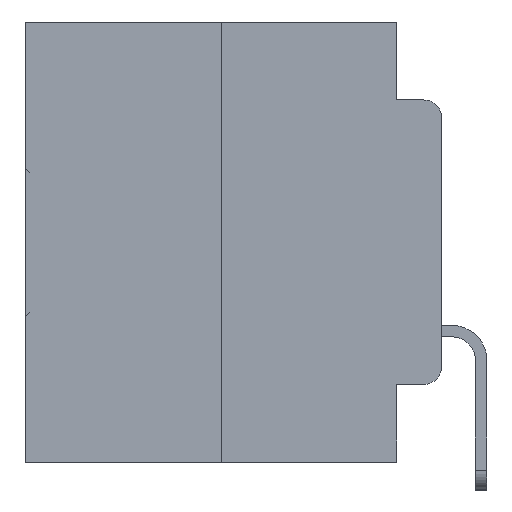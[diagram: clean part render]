
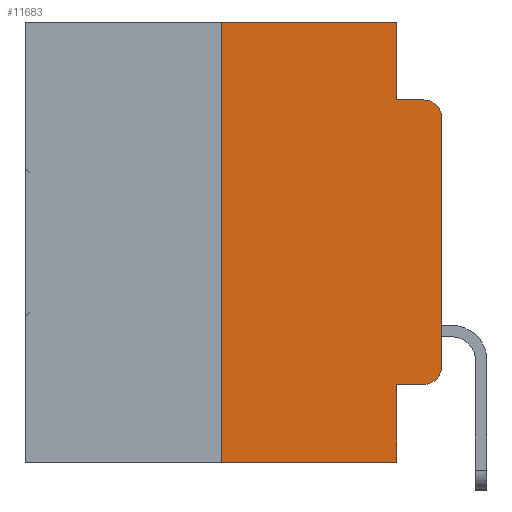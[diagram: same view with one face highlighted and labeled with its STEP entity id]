
A CAD part, left-side view. The second image highlights one B-rep face of the part: STEP entity #11683.
In plain terms, the highlighted planar face has unit normal (-1, 0, 0).
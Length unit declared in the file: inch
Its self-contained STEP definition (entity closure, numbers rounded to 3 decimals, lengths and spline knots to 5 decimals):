
#506 = CARTESIAN_POINT ( 'NONE',  ( 0., 0.473, -0.5 ) ) ;
#523 = LINE ( 'NONE', #14726, #13903 ) ;
#808 = CARTESIAN_POINT ( 'NONE',  ( 0., 0.051, -0.4115 ) ) ;
#1517 = CARTESIAN_POINT ( 'NONE',  ( 0., 0.473, 0. ) ) ;
#1550 = EDGE_CURVE ( 'NONE', #27723, #16165, #23982, .T. ) ;
#2521 = LINE ( 'NONE', #28439, #27292 ) ;
#3040 = CARTESIAN_POINT ( 'NONE',  ( 0., 0.051, 0. ) ) ;
#3444 = AXIS2_PLACEMENT_3D ( 'NONE', #1517, #19579, #4338 ) ;
#4338 = DIRECTION ( 'NONE',  ( 0., 0., -1. ) ) ;
#4409 = EDGE_LOOP ( 'NONE', ( #30576, #19176, #9866, #19543, #31645, #8665, #29174, #15020, #27448, #17326 ) ) ;
#4713 = VERTEX_POINT ( 'NONE', #7972 ) ;
#4995 = CARTESIAN_POINT ( 'NONE',  ( 0., 0.02, -0.1085 ) ) ;
#5951 = CARTESIAN_POINT ( 'NONE',  ( 0., 0., -0.1085 ) ) ;
#7069 = VERTEX_POINT ( 'NONE', #9125 ) ;
#7181 = DIRECTION ( 'NONE',  ( 0., 0., -1. ) ) ;
#7466 = CIRCLE ( 'NONE', #23512, 0.02 ) ;
#7744 = DIRECTION ( 'NONE',  ( 0., 0., -1. ) ) ;
#7972 = CARTESIAN_POINT ( 'NONE',  ( 0., 0.25, -0.5 ) ) ;
#8665 = ORIENTED_EDGE ( 'NONE', *, *, #12563, .F. ) ;
#9125 = CARTESIAN_POINT ( 'NONE',  ( 0., 0.051, -0.0885 ) ) ;
#9246 = DIRECTION ( 'NONE',  ( 0., -1., 0. ) ) ;
#9646 = VERTEX_POINT ( 'NONE', #808 ) ;
#9866 = ORIENTED_EDGE ( 'NONE', *, *, #18509, .F. ) ;
#11180 = VECTOR ( 'NONE', #24997, 39.37008 ) ;
#11683 = ADVANCED_FACE ( 'NONE', ( #27561 ), #26423, .F. ) ;
#11932 = LINE ( 'NONE', #506, #29934 ) ;
#12384 = CARTESIAN_POINT ( 'NONE',  ( 0., 0.051, -0.0885 ) ) ;
#12563 = EDGE_CURVE ( 'NONE', #4713, #16978, #14707, .T. ) ;
#12642 = CARTESIAN_POINT ( 'NONE',  ( 0., 0.02, -0.3915 ) ) ;
#13329 = CARTESIAN_POINT ( 'NONE',  ( 0., 0., -0.3915 ) ) ;
#13543 = VERTEX_POINT ( 'NONE', #19610 ) ;
#13674 = CIRCLE ( 'NONE', #15097, 0.02 ) ;
#13903 = VECTOR ( 'NONE', #17190, 39.37008 ) ;
#14136 = LINE ( 'NONE', #12384, #31931 ) ;
#14707 = LINE ( 'NONE', #27956, #26469 ) ;
#14726 = CARTESIAN_POINT ( 'NONE',  ( 0., 0.473, 0. ) ) ;
#14885 = DIRECTION ( 'NONE',  ( 0., -1., 0. ) ) ;
#14890 = CARTESIAN_POINT ( 'NONE',  ( 0., 0.051, 0. ) ) ;
#15020 = ORIENTED_EDGE ( 'NONE', *, *, #30381, .F. ) ;
#15097 = AXIS2_PLACEMENT_3D ( 'NONE', #4995, #22463, #7744 ) ;
#15130 = DIRECTION ( 'NONE',  ( 0., 0., -1. ) ) ;
#16165 = VERTEX_POINT ( 'NONE', #5951 ) ;
#16978 = VERTEX_POINT ( 'NONE', #28145 ) ;
#17190 = DIRECTION ( 'NONE',  ( 0., -1., 0. ) ) ;
#17326 = ORIENTED_EDGE ( 'NONE', *, *, #29039, .T. ) ;
#17896 = VERTEX_POINT ( 'NONE', #31397 ) ;
#18509 = EDGE_CURVE ( 'NONE', #7069, #19361, #14136, .T. ) ;
#19176 = ORIENTED_EDGE ( 'NONE', *, *, #22638, .T. ) ;
#19361 = VERTEX_POINT ( 'NONE', #31208 ) ;
#19543 = ORIENTED_EDGE ( 'NONE', *, *, #29808, .F. ) ;
#19579 = DIRECTION ( 'NONE',  ( 1., 0., 0. ) ) ;
#19610 = CARTESIAN_POINT ( 'NONE',  ( 0., 0.02, -0.4115 ) ) ;
#19657 = VERTEX_POINT ( 'NONE', #21021 ) ;
#20865 = DIRECTION ( 'NONE',  ( 0., 0., -1. ) ) ;
#21021 = CARTESIAN_POINT ( 'NONE',  ( 0., 0.051, -0.5 ) ) ;
#21140 = DIRECTION ( 'NONE',  ( 0., -1., 0. ) ) ;
#22463 = DIRECTION ( 'NONE',  ( -1., 0., 0. ) ) ;
#22638 = EDGE_CURVE ( 'NONE', #16165, #19361, #13674, .T. ) ;
#23369 = LINE ( 'NONE', #3040, #28646 ) ;
#23512 = AXIS2_PLACEMENT_3D ( 'NONE', #12642, #29044, #15130 ) ;
#23982 = LINE ( 'NONE', #24961, #11180 ) ;
#24854 = LINE ( 'NONE', #14890, #30791 ) ;
#24961 = CARTESIAN_POINT ( 'NONE',  ( 0., 0., 0. ) ) ;
#24997 = DIRECTION ( 'NONE',  ( 0., 0., 1. ) ) ;
#25490 = EDGE_CURVE ( 'NONE', #9646, #13543, #2521, .T. ) ;
#26423 = PLANE ( 'NONE',  #3444 ) ;
#26469 = VECTOR ( 'NONE', #30216, 39.37008 ) ;
#27292 = VECTOR ( 'NONE', #9246, 39.37008 ) ;
#27448 = ORIENTED_EDGE ( 'NONE', *, *, #25490, .T. ) ;
#27561 = FACE_OUTER_BOUND ( 'NONE', #4409, .T. ) ;
#27723 = VERTEX_POINT ( 'NONE', #13329 ) ;
#27956 = CARTESIAN_POINT ( 'NONE',  ( 0., 0.25, 0. ) ) ;
#28145 = CARTESIAN_POINT ( 'NONE',  ( 0., 0.25, 0. ) ) ;
#28229 = EDGE_CURVE ( 'NONE', #16978, #17896, #523, .T. ) ;
#28439 = CARTESIAN_POINT ( 'NONE',  ( 0., 0.051, -0.4115 ) ) ;
#28600 = EDGE_CURVE ( 'NONE', #4713, #19657, #11932, .T. ) ;
#28646 = VECTOR ( 'NONE', #20865, 39.37008 ) ;
#29039 = EDGE_CURVE ( 'NONE', #13543, #27723, #7466, .T. ) ;
#29044 = DIRECTION ( 'NONE',  ( -1., 0., 0. ) ) ;
#29174 = ORIENTED_EDGE ( 'NONE', *, *, #28600, .T. ) ;
#29808 = EDGE_CURVE ( 'NONE', #17896, #7069, #24854, .T. ) ;
#29934 = VECTOR ( 'NONE', #21140, 39.37008 ) ;
#30216 = DIRECTION ( 'NONE',  ( 0., 0., 1. ) ) ;
#30381 = EDGE_CURVE ( 'NONE', #9646, #19657, #23369, .T. ) ;
#30576 = ORIENTED_EDGE ( 'NONE', *, *, #1550, .T. ) ;
#30791 = VECTOR ( 'NONE', #7181, 39.37008 ) ;
#31208 = CARTESIAN_POINT ( 'NONE',  ( 0., 0.02, -0.0885 ) ) ;
#31397 = CARTESIAN_POINT ( 'NONE',  ( 0., 0.051, 0. ) ) ;
#31645 = ORIENTED_EDGE ( 'NONE', *, *, #28229, .F. ) ;
#31931 = VECTOR ( 'NONE', #14885, 39.37008 ) ;
